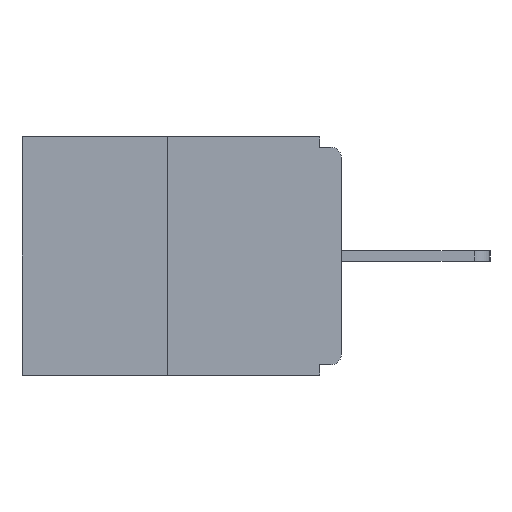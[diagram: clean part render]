
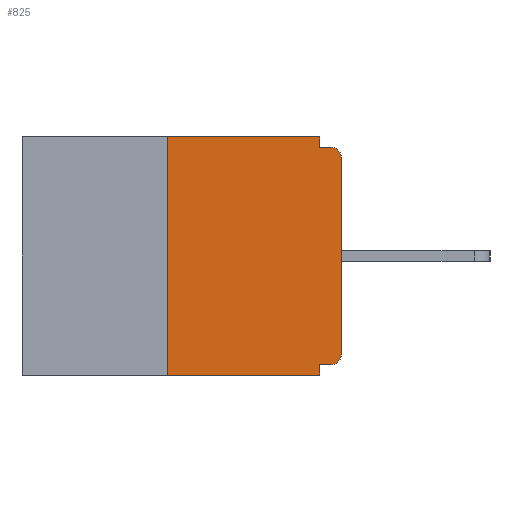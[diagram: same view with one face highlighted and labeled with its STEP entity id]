
A CAD part, left-side view. The second image highlights one B-rep face of the part: STEP entity #825.
In plain terms, the highlighted planar face has unit normal (-1, 0, 0).
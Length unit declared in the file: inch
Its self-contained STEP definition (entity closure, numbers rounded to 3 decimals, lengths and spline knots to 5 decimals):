
#72 = LINE ( 'NONE', #3270, #3363 ) ;
#127 = CARTESIAN_POINT ( 'NONE',  ( 0., 0.031, -0.015 ) ) ;
#148 = VERTEX_POINT ( 'NONE', #5324 ) ;
#208 = ORIENTED_EDGE ( 'NONE', *, *, #12135, .T. ) ;
#241 = AXIS2_PLACEMENT_3D ( 'NONE', #12317, #6648, #13267 ) ;
#479 = EDGE_CURVE ( 'NONE', #1583, #2248, #9553, .T. ) ;
#527 = AXIS2_PLACEMENT_3D ( 'NONE', #3789, #1771, #2378 ) ;
#637 = VERTEX_POINT ( 'NONE', #12910 ) ;
#825 = ADVANCED_FACE ( 'NONE', ( #6071 ), #3740, .F. ) ;
#1235 = ORIENTED_EDGE ( 'NONE', *, *, #11206, .T. ) ;
#1397 = VECTOR ( 'NONE', #10948, 39.37008 ) ;
#1525 = DIRECTION ( 'NONE',  ( 0., 0., 1. ) ) ;
#1583 = VERTEX_POINT ( 'NONE', #13306 ) ;
#1650 = CIRCLE ( 'NONE', #241, 0.015 ) ;
#1723 = CARTESIAN_POINT ( 'NONE',  ( 0., 0., -0.328 ) ) ;
#1771 = DIRECTION ( 'NONE',  ( 1., 0., 0. ) ) ;
#1993 = DIRECTION ( 'NONE',  ( 0., -1., 0. ) ) ;
#2014 = CARTESIAN_POINT ( 'NONE',  ( 0., 0., -0.015 ) ) ;
#2225 = ORIENTED_EDGE ( 'NONE', *, *, #9335, .F. ) ;
#2248 = VERTEX_POINT ( 'NONE', #12513 ) ;
#2281 = ORIENTED_EDGE ( 'NONE', *, *, #2337, .T. ) ;
#2337 = EDGE_CURVE ( 'NONE', #7692, #1583, #13281, .T. ) ;
#2378 = DIRECTION ( 'NONE',  ( 0., 0., -1. ) ) ;
#2448 = DIRECTION ( 'NONE',  ( 0., 0., -1. ) ) ;
#2481 = CARTESIAN_POINT ( 'NONE',  ( 0., 0.031, 0. ) ) ;
#2515 = ORIENTED_EDGE ( 'NONE', *, *, #11816, .F. ) ;
#2555 = CARTESIAN_POINT ( 'NONE',  ( 0., 0.25, 0. ) ) ;
#2805 = VERTEX_POINT ( 'NONE', #13141 ) ;
#2920 = EDGE_LOOP ( 'NONE', ( #2515, #5198, #1235, #5227, #4394, #208, #2281, #6246, #6461, #2225 ) ) ;
#2954 = DIRECTION ( 'NONE',  ( 0., -1., 0. ) ) ;
#3229 = LINE ( 'NONE', #2014, #8442 ) ;
#3270 = CARTESIAN_POINT ( 'NONE',  ( 0., 0.46, -0.343 ) ) ;
#3363 = VECTOR ( 'NONE', #4438, 39.37008 ) ;
#3740 = PLANE ( 'NONE',  #527 ) ;
#3746 = DIRECTION ( 'NONE',  ( 0., 0., 1. ) ) ;
#3789 = CARTESIAN_POINT ( 'NONE',  ( 0., 0.46, 0. ) ) ;
#4249 = VECTOR ( 'NONE', #2954, 39.37008 ) ;
#4394 = ORIENTED_EDGE ( 'NONE', *, *, #6581, .F. ) ;
#4395 = VECTOR ( 'NONE', #3746, 39.37008 ) ;
#4438 = DIRECTION ( 'NONE',  ( 0., -1., 0. ) ) ;
#4560 = LINE ( 'NONE', #1723, #1397 ) ;
#4973 = AXIS2_PLACEMENT_3D ( 'NONE', #11463, #10296, #11339 ) ;
#5089 = CARTESIAN_POINT ( 'NONE',  ( 0., 0.031, -0.328 ) ) ;
#5198 = ORIENTED_EDGE ( 'NONE', *, *, #13097, .F. ) ;
#5227 = ORIENTED_EDGE ( 'NONE', *, *, #9953, .F. ) ;
#5324 = CARTESIAN_POINT ( 'NONE',  ( 0., 0.25, -0.343 ) ) ;
#5775 = VERTEX_POINT ( 'NONE', #5089 ) ;
#5821 = LINE ( 'NONE', #7038, #13125 ) ;
#6071 = FACE_OUTER_BOUND ( 'NONE', #2920, .T. ) ;
#6246 = ORIENTED_EDGE ( 'NONE', *, *, #479, .T. ) ;
#6290 = VERTEX_POINT ( 'NONE', #127 ) ;
#6461 = ORIENTED_EDGE ( 'NONE', *, *, #9410, .F. ) ;
#6581 = EDGE_CURVE ( 'NONE', #10608, #5775, #4560, .T. ) ;
#6648 = DIRECTION ( 'NONE',  ( -1., 0., 0. ) ) ;
#6804 = CARTESIAN_POINT ( 'NONE',  ( 0., 0.015, -0.328 ) ) ;
#7038 = CARTESIAN_POINT ( 'NONE',  ( 0., 0.031, -0.343 ) ) ;
#7692 = VERTEX_POINT ( 'NONE', #12193 ) ;
#8351 = CARTESIAN_POINT ( 'NONE',  ( 0., 0., 0. ) ) ;
#8442 = VECTOR ( 'NONE', #1993, 39.37008 ) ;
#9334 = LINE ( 'NONE', #2481, #12098 ) ;
#9335 = EDGE_CURVE ( 'NONE', #637, #6290, #9334, .T. ) ;
#9410 = EDGE_CURVE ( 'NONE', #6290, #2248, #3229, .T. ) ;
#9553 = CIRCLE ( 'NONE', #4973, 0.015 ) ;
#9953 = EDGE_CURVE ( 'NONE', #5775, #2805, #5821, .T. ) ;
#10296 = DIRECTION ( 'NONE',  ( -1., 0., 0. ) ) ;
#10608 = VERTEX_POINT ( 'NONE', #6804 ) ;
#10799 = VECTOR ( 'NONE', #1525, 39.37008 ) ;
#10948 = DIRECTION ( 'NONE',  ( 0., 1., 0. ) ) ;
#11206 = EDGE_CURVE ( 'NONE', #148, #2805, #72, .T. ) ;
#11339 = DIRECTION ( 'NONE',  ( 0., 0., -1. ) ) ;
#11463 = CARTESIAN_POINT ( 'NONE',  ( 0., 0.015, -0.03 ) ) ;
#11629 = VERTEX_POINT ( 'NONE', #12710 ) ;
#11816 = EDGE_CURVE ( 'NONE', #11629, #637, #12037, .T. ) ;
#11917 = CARTESIAN_POINT ( 'NONE',  ( 0., 0.46, 0. ) ) ;
#12037 = LINE ( 'NONE', #11917, #4249 ) ;
#12098 = VECTOR ( 'NONE', #2448, 39.37008 ) ;
#12135 = EDGE_CURVE ( 'NONE', #10608, #7692, #1650, .T. ) ;
#12193 = CARTESIAN_POINT ( 'NONE',  ( 0., 0., -0.313 ) ) ;
#12317 = CARTESIAN_POINT ( 'NONE',  ( 0., 0.015, -0.313 ) ) ;
#12460 = LINE ( 'NONE', #2555, #4395 ) ;
#12513 = CARTESIAN_POINT ( 'NONE',  ( 0., 0.015, -0.015 ) ) ;
#12710 = CARTESIAN_POINT ( 'NONE',  ( 0., 0.25, 0. ) ) ;
#12738 = DIRECTION ( 'NONE',  ( 0., 0., -1. ) ) ;
#12910 = CARTESIAN_POINT ( 'NONE',  ( 0., 0.031, 0. ) ) ;
#13097 = EDGE_CURVE ( 'NONE', #148, #11629, #12460, .T. ) ;
#13125 = VECTOR ( 'NONE', #12738, 39.37008 ) ;
#13141 = CARTESIAN_POINT ( 'NONE',  ( 0., 0.031, -0.343 ) ) ;
#13267 = DIRECTION ( 'NONE',  ( 0., 0., -1. ) ) ;
#13281 = LINE ( 'NONE', #8351, #10799 ) ;
#13306 = CARTESIAN_POINT ( 'NONE',  ( 0., 0., -0.03 ) ) ;
